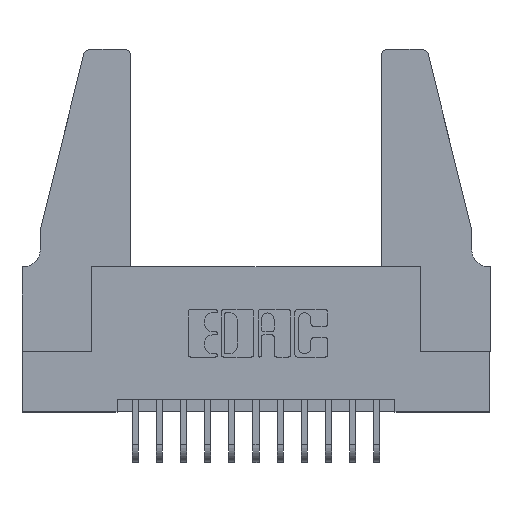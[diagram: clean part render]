
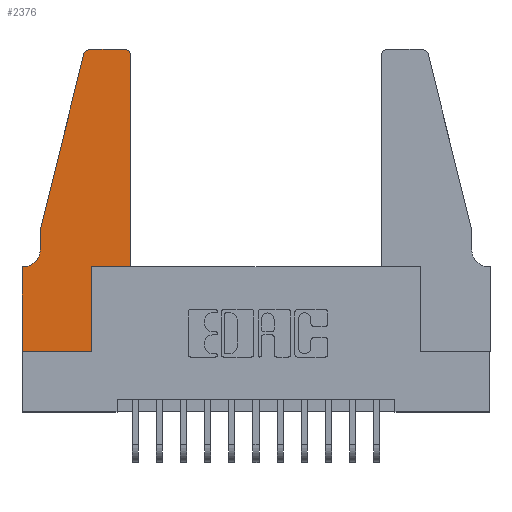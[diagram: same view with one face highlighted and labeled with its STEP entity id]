
A CAD part, top view. The second image highlights one B-rep face of the part: STEP entity #2376.
In plain terms, the highlighted planar face has unit normal (0, 0, 1).
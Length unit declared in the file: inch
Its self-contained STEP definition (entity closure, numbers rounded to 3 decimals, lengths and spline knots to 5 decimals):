
#17 = EDGE_CURVE ( 'NONE', #6548, #12867, #15363, .T. ) ;
#38 = VECTOR ( 'NONE', #5539, 39.37008 ) ;
#323 = DIRECTION ( 'NONE',  ( -0.239, -0.971, 0. ) ) ;
#333 = LINE ( 'NONE', #10222, #12581 ) ;
#522 = DIRECTION ( 'NONE',  ( 0., 1., 0. ) ) ;
#829 = EDGE_CURVE ( 'NONE', #2587, #11338, #12521, .T. ) ;
#833 = CARTESIAN_POINT ( 'NONE',  ( 0.4205, 1.25, 0.37 ) ) ;
#1084 = ORIENTED_EDGE ( 'NONE', *, *, #13813, .T. ) ;
#1389 = EDGE_CURVE ( 'NONE', #8625, #12034, #16157, .T. ) ;
#1405 = DIRECTION ( 'NONE',  ( 0., 0., 1. ) ) ;
#1674 = LINE ( 'NONE', #4310, #38 ) ;
#1690 = EDGE_CURVE ( 'NONE', #11338, #6548, #8950, .T. ) ;
#1749 = ORIENTED_EDGE ( 'NONE', *, *, #6547, .T. ) ;
#2154 = DIRECTION ( 'NONE',  ( 0., 0., 1. ) ) ;
#2376 = ADVANCED_FACE ( 'NONE', ( #5731 ), #7844, .T. ) ;
#2455 = VECTOR ( 'NONE', #6499, 39.37008 ) ;
#2497 = CARTESIAN_POINT ( 'NONE',  ( 0.4505, 0.35, 0.37 ) ) ;
#2558 = LINE ( 'NONE', #7178, #8200 ) ;
#2587 = VERTEX_POINT ( 'NONE', #15199 ) ;
#2656 = LINE ( 'NONE', #10301, #2455 ) ;
#2770 = ORIENTED_EDGE ( 'NONE', *, *, #5376, .T. ) ;
#2823 = CARTESIAN_POINT ( 'NONE',  ( 0.0755, 0.35, 0.37 ) ) ;
#3157 = VERTEX_POINT ( 'NONE', #15303 ) ;
#3160 = CARTESIAN_POINT ( 'NONE',  ( 0.4505, 0.35, 0.37 ) ) ;
#3222 = LINE ( 'NONE', #5687, #6248 ) ;
#3539 = ORIENTED_EDGE ( 'NONE', *, *, #17, .T. ) ;
#3575 = AXIS2_PLACEMENT_3D ( 'NONE', #11601, #1405, #15555 ) ;
#3831 = EDGE_CURVE ( 'NONE', #12867, #15460, #2656, .T. ) ;
#3984 = CARTESIAN_POINT ( 'NONE',  ( 0., 0., 0.37 ) ) ;
#4179 = CARTESIAN_POINT ( 'NONE',  ( 0.2865, 0.35, 0.37 ) ) ;
#4310 = CARTESIAN_POINT ( 'NONE',  ( 0., 0., 0.37 ) ) ;
#4528 = DIRECTION ( 'NONE',  ( 1., 0., 0. ) ) ;
#4726 = DIRECTION ( 'NONE',  ( -1., 0., 0. ) ) ;
#4780 = EDGE_CURVE ( 'NONE', #4838, #8529, #3222, .T. ) ;
#4838 = VERTEX_POINT ( 'NONE', #15825 ) ;
#5137 = CARTESIAN_POINT ( 'NONE',  ( 0.284, 1.22, 0.37 ) ) ;
#5376 = EDGE_CURVE ( 'NONE', #15460, #4838, #15835, .T. ) ;
#5539 = DIRECTION ( 'NONE',  ( 1., 0., 0. ) ) ;
#5687 = CARTESIAN_POINT ( 'NONE',  ( 0.0755, 0.5, 0.37 ) ) ;
#5731 = FACE_OUTER_BOUND ( 'NONE', #9943, .T. ) ;
#5975 = LINE ( 'NONE', #4179, #13166 ) ;
#6148 = CIRCLE ( 'NONE', #11703, 0.07 ) ;
#6248 = VECTOR ( 'NONE', #323, 39.37008 ) ;
#6262 = ORIENTED_EDGE ( 'NONE', *, *, #8366, .T. ) ;
#6411 = CARTESIAN_POINT ( 'NONE',  ( 0.4505, 1.22, 0.37 ) ) ;
#6499 = DIRECTION ( 'NONE',  ( -1., 0., 0. ) ) ;
#6541 = VECTOR ( 'NONE', #9069, 39.37008 ) ;
#6547 = EDGE_CURVE ( 'NONE', #12034, #6990, #333, .T. ) ;
#6548 = VERTEX_POINT ( 'NONE', #6411 ) ;
#6707 = ORIENTED_EDGE ( 'NONE', *, *, #829, .T. ) ;
#6854 = ORIENTED_EDGE ( 'NONE', *, *, #1690, .T. ) ;
#6990 = VERTEX_POINT ( 'NONE', #3984 ) ;
#7070 = CARTESIAN_POINT ( 'NONE',  ( 0., 0.35, 0.37 ) ) ;
#7178 = CARTESIAN_POINT ( 'NONE',  ( 0.0755, 0.5, 0.37 ) ) ;
#7816 = ORIENTED_EDGE ( 'NONE', *, *, #4780, .T. ) ;
#7844 = PLANE ( 'NONE',  #3575 ) ;
#7866 = AXIS2_PLACEMENT_3D ( 'NONE', #9638, #2154, #4528 ) ;
#7881 = ORIENTED_EDGE ( 'NONE', *, *, #1389, .T. ) ;
#8200 = VECTOR ( 'NONE', #9494, 39.37008 ) ;
#8260 = CARTESIAN_POINT ( 'NONE',  ( 0.4505, 0.35, 0.37 ) ) ;
#8366 = EDGE_CURVE ( 'NONE', #6990, #12280, #1674, .T. ) ;
#8529 = VERTEX_POINT ( 'NONE', #16113 ) ;
#8625 = VERTEX_POINT ( 'NONE', #15203 ) ;
#8843 = DIRECTION ( 'NONE',  ( 1., 0., 0. ) ) ;
#8950 = LINE ( 'NONE', #8260, #15751 ) ;
#9069 = DIRECTION ( 'NONE',  ( 1., 0., 0. ) ) ;
#9166 = DIRECTION ( 'NONE',  ( 0., 1., 0. ) ) ;
#9494 = DIRECTION ( 'NONE',  ( 0., -1., 0. ) ) ;
#9638 = CARTESIAN_POINT ( 'NONE',  ( 0.4205, 1.22, 0.37 ) ) ;
#9783 = CARTESIAN_POINT ( 'NONE',  ( 0.0055, 0.42, 0.37 ) ) ;
#9937 = DIRECTION ( 'NONE',  ( 0., 0., -1. ) ) ;
#9943 = EDGE_LOOP ( 'NONE', ( #10598, #2770, #7816, #15701, #1084, #7881, #1749, #6262, #14133, #6707, #6854, #3539 ) ) ;
#10187 = DIRECTION ( 'NONE',  ( 0., 0., 1. ) ) ;
#10222 = CARTESIAN_POINT ( 'NONE',  ( 0., 0., 0.37 ) ) ;
#10301 = CARTESIAN_POINT ( 'NONE',  ( 0.2605, 1.25, 0.37 ) ) ;
#10598 = ORIENTED_EDGE ( 'NONE', *, *, #3831, .T. ) ;
#11165 = VECTOR ( 'NONE', #11821, 39.37008 ) ;
#11338 = VERTEX_POINT ( 'NONE', #3160 ) ;
#11601 = CARTESIAN_POINT ( 'NONE',  ( 0., 0.35, 0.37 ) ) ;
#11703 = AXIS2_PLACEMENT_3D ( 'NONE', #9783, #9937, #4726 ) ;
#11821 = DIRECTION ( 'NONE',  ( -1., 0., 0. ) ) ;
#12011 = EDGE_CURVE ( 'NONE', #8529, #3157, #2558, .T. ) ;
#12034 = VERTEX_POINT ( 'NONE', #7070 ) ;
#12280 = VERTEX_POINT ( 'NONE', #15235 ) ;
#12521 = LINE ( 'NONE', #2497, #6541 ) ;
#12581 = VECTOR ( 'NONE', #13499, 39.37008 ) ;
#12867 = VERTEX_POINT ( 'NONE', #833 ) ;
#13166 = VECTOR ( 'NONE', #9166, 39.37008 ) ;
#13499 = DIRECTION ( 'NONE',  ( 0., -1., 0. ) ) ;
#13813 = EDGE_CURVE ( 'NONE', #3157, #8625, #6148, .T. ) ;
#14133 = ORIENTED_EDGE ( 'NONE', *, *, #15516, .T. ) ;
#14202 = CARTESIAN_POINT ( 'NONE',  ( 0.284, 1.25, 0.37 ) ) ;
#15199 = CARTESIAN_POINT ( 'NONE',  ( 0.2865, 0.35, 0.37 ) ) ;
#15203 = CARTESIAN_POINT ( 'NONE',  ( 0.0055, 0.35, 0.37 ) ) ;
#15235 = CARTESIAN_POINT ( 'NONE',  ( 0.2865, 0., 0.37 ) ) ;
#15303 = CARTESIAN_POINT ( 'NONE',  ( 0.0755, 0.42, 0.37 ) ) ;
#15363 = CIRCLE ( 'NONE', #7866, 0.03 ) ;
#15423 = AXIS2_PLACEMENT_3D ( 'NONE', #5137, #10187, #8843 ) ;
#15460 = VERTEX_POINT ( 'NONE', #14202 ) ;
#15516 = EDGE_CURVE ( 'NONE', #12280, #2587, #5975, .T. ) ;
#15555 = DIRECTION ( 'NONE',  ( 1., 0., 0. ) ) ;
#15701 = ORIENTED_EDGE ( 'NONE', *, *, #12011, .T. ) ;
#15751 = VECTOR ( 'NONE', #522, 39.37008 ) ;
#15825 = CARTESIAN_POINT ( 'NONE',  ( 0.25487, 1.22718, 0.37 ) ) ;
#15835 = CIRCLE ( 'NONE', #15423, 0.03 ) ;
#16113 = CARTESIAN_POINT ( 'NONE',  ( 0.0755, 0.5, 0.37 ) ) ;
#16157 = LINE ( 'NONE', #2823, #11165 ) ;
